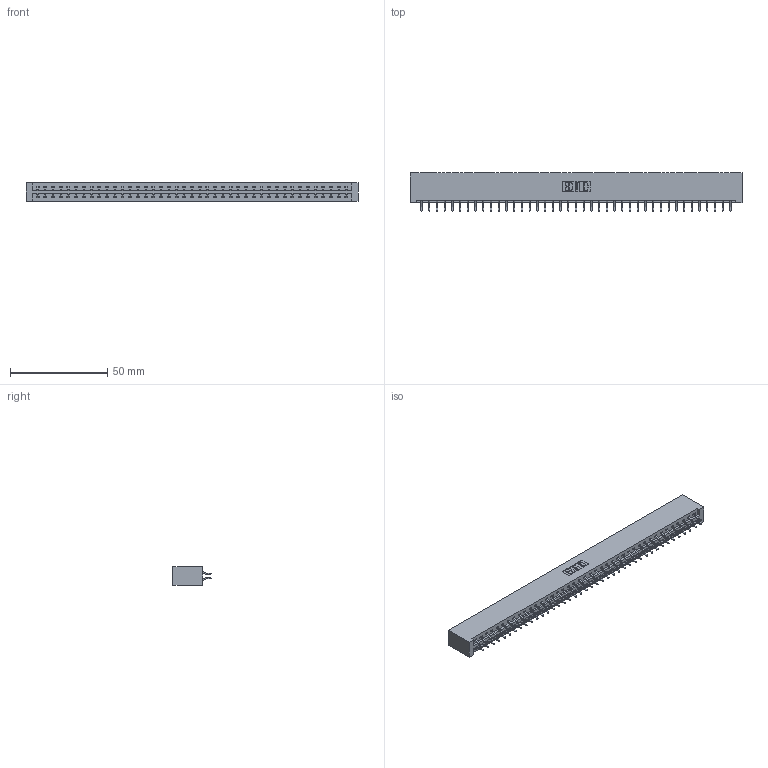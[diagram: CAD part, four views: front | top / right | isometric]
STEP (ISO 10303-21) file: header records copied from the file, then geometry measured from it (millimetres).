
FILE_DESCRIPTION (( 'STEP AP203' ), '1' );
FILE_NAME ('337-082-556-201.STEP', '2019-10-10T13:19:52', ( '' ), ( '' ), 'SwSTEP 2.0', 'SolidWorks 2016', '' );
FILE_SCHEMA (( 'CONFIG_CONTROL_DESIGN' ));
Length unit declared in the file: inch
Products named in the file (3): 345-292-001_556 Tail; 337-082-556-201; 337 Part_No Mounting Lugs
Assembly tree (83 placements, depth 2):
  337-082-556-201
    337 Part_No Mounting Lugs
    345-292-001_556 Tail  x82
Bounding box: 170.33 x 19.57 x 9.4 mm (x, y, z)
Volume: 18695.2 mm3; surface area: 21094.8 mm2
Topology: 83 solids, 83 shells, 5026 faces, 14965 edges, 9866 vertices
Faces by surface type: plane 3510, cylinder 1516
Entity records: 31861 total; most frequent: CARTESIAN_POINT 5382, ORIENTED_EDGE 5306, DIRECTION 4561, EDGE_CURVE 2653, VECTOR 2525, LINE 2525, VERTEX_POINT 1766, AXIS2_PLACEMENT_3D 1018
